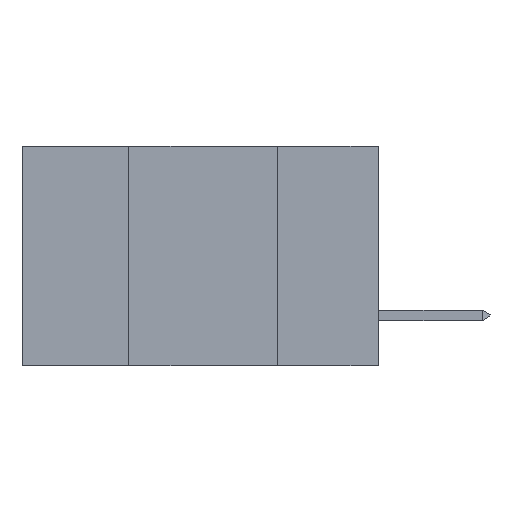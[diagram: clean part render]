
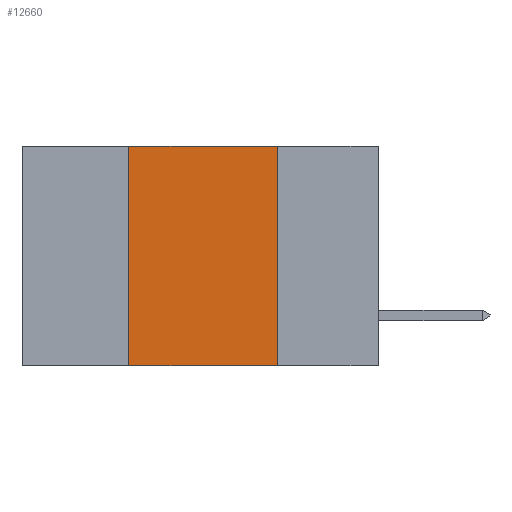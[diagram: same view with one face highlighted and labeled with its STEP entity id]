
A CAD part, left-side view. The second image highlights one B-rep face of the part: STEP entity #12660.
In plain terms, the highlighted planar face has unit normal (-1, 0, 0).
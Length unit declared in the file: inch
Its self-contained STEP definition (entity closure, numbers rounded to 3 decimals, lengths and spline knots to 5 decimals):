
#1362 = PLANE ( 'NONE',  #19734 ) ;
#2189 = EDGE_CURVE ( 'NONE', #5243, #6610, #2295, .T. ) ;
#2295 = LINE ( 'NONE', #5796, #12746 ) ;
#4313 = VECTOR ( 'NONE', #12219, 39.37008 ) ;
#4446 = ORIENTED_EDGE ( 'NONE', *, *, #9769, .T. ) ;
#4637 = LINE ( 'NONE', #9031, #10172 ) ;
#5243 = VERTEX_POINT ( 'NONE', #11712 ) ;
#5796 = CARTESIAN_POINT ( 'NONE',  ( 0., 0.6, 0. ) ) ;
#5828 = DIRECTION ( 'NONE',  ( 1., 0., 0. ) ) ;
#6034 = FACE_OUTER_BOUND ( 'NONE', #17535, .T. ) ;
#6610 = VERTEX_POINT ( 'NONE', #17741 ) ;
#6906 = LINE ( 'NONE', #14719, #14771 ) ;
#7194 = LINE ( 'NONE', #15223, #4313 ) ;
#8115 = ORIENTED_EDGE ( 'NONE', *, *, #2189, .F. ) ;
#9031 = CARTESIAN_POINT ( 'NONE',  ( 0., 0.17, -0.37 ) ) ;
#9614 = ORIENTED_EDGE ( 'NONE', *, *, #14328, .F. ) ;
#9769 = EDGE_CURVE ( 'NONE', #15177, #16952, #7194, .T. ) ;
#10172 = VECTOR ( 'NONE', #20462, 39.37008 ) ;
#10871 = DIRECTION ( 'NONE',  ( 0., 0., -1. ) ) ;
#11712 = CARTESIAN_POINT ( 'NONE',  ( 0., 0.42, 0. ) ) ;
#12186 = ORIENTED_EDGE ( 'NONE', *, *, #19697, .F. ) ;
#12219 = DIRECTION ( 'NONE',  ( 0., -1., 0. ) ) ;
#12660 = ADVANCED_FACE ( 'NONE', ( #6034 ), #1362, .F. ) ;
#12746 = VECTOR ( 'NONE', #17251, 39.37008 ) ;
#13951 = CARTESIAN_POINT ( 'NONE',  ( 0., 0.6, 0. ) ) ;
#14076 = CARTESIAN_POINT ( 'NONE',  ( 0., 0.42, -0.37 ) ) ;
#14328 = EDGE_CURVE ( 'NONE', #6610, #16952, #4637, .T. ) ;
#14719 = CARTESIAN_POINT ( 'NONE',  ( 0., 0.42, -0.37 ) ) ;
#14771 = VECTOR ( 'NONE', #19643, 39.37008 ) ;
#15177 = VERTEX_POINT ( 'NONE', #14076 ) ;
#15223 = CARTESIAN_POINT ( 'NONE',  ( 0., 0.6, -0.37 ) ) ;
#16952 = VERTEX_POINT ( 'NONE', #17519 ) ;
#17251 = DIRECTION ( 'NONE',  ( 0., -1., 0. ) ) ;
#17519 = CARTESIAN_POINT ( 'NONE',  ( 0., 0.17, -0.37 ) ) ;
#17535 = EDGE_LOOP ( 'NONE', ( #9614, #8115, #12186, #4446 ) ) ;
#17741 = CARTESIAN_POINT ( 'NONE',  ( 0., 0.17, 0. ) ) ;
#19643 = DIRECTION ( 'NONE',  ( 0., 0., 1. ) ) ;
#19697 = EDGE_CURVE ( 'NONE', #15177, #5243, #6906, .T. ) ;
#19734 = AXIS2_PLACEMENT_3D ( 'NONE', #13951, #5828, #10871 ) ;
#20462 = DIRECTION ( 'NONE',  ( 0., 0., -1. ) ) ;
